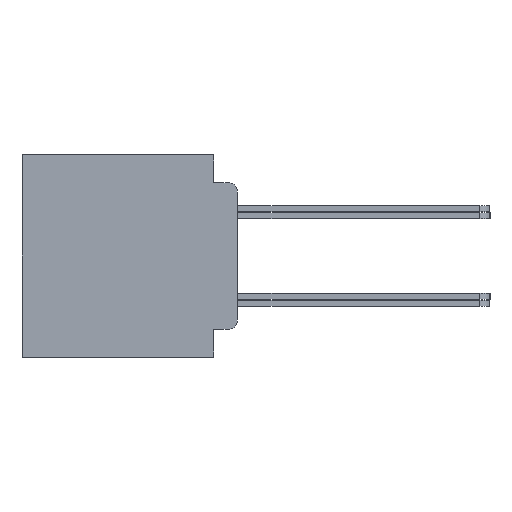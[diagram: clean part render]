
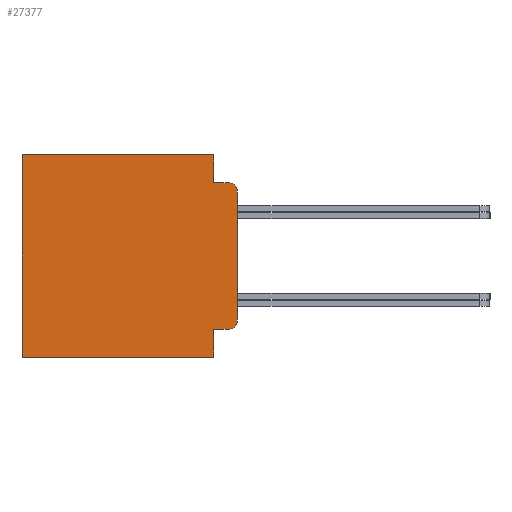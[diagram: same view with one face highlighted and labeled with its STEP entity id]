
A CAD part, left-side view. The second image highlights one B-rep face of the part: STEP entity #27377.
In plain terms, the highlighted planar face has unit normal (-1, 0, 0).
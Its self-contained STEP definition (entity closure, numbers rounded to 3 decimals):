
#7 = VECTOR ( 'NONE', #24448, 1000. ) ;
#81 = CARTESIAN_POINT ( 'NONE',  ( -67.462, 1.295, -3.975 ) ) ;
#483 = VECTOR ( 'NONE', #7830, 1000. ) ;
#488 = ORIENTED_EDGE ( 'NONE', *, *, #22660, .F. ) ;
#946 = CARTESIAN_POINT ( 'NONE',  ( -67.462, 1.295, 3.975 ) ) ;
#1349 = VERTEX_POINT ( 'NONE', #946 ) ;
#1494 = CARTESIAN_POINT ( 'NONE',  ( -67.462, 0., 3.467 ) ) ;
#2006 = EDGE_CURVE ( 'NONE', #25729, #3669, #11912, .T. ) ;
#2063 = LINE ( 'NONE', #21804, #12012 ) ;
#2272 = CARTESIAN_POINT ( 'NONE',  ( -67.462, 11.684, 5.486 ) ) ;
#2387 = AXIS2_PLACEMENT_3D ( 'NONE', #2771, #26645, #26544 ) ;
#2401 = DIRECTION ( 'NONE',  ( 0., 1., 0. ) ) ;
#2612 = VECTOR ( 'NONE', #22150, 1000. ) ;
#2771 = CARTESIAN_POINT ( 'NONE',  ( -67.462, 0., -5.486 ) ) ;
#2920 = ORIENTED_EDGE ( 'NONE', *, *, #2006, .F. ) ;
#3669 = VERTEX_POINT ( 'NONE', #18018 ) ;
#5300 = LINE ( 'NONE', #18003, #5620 ) ;
#5378 = ORIENTED_EDGE ( 'NONE', *, *, #16718, .F. ) ;
#5521 = CARTESIAN_POINT ( 'NONE',  ( -67.462, 0., 5.486 ) ) ;
#5620 = VECTOR ( 'NONE', #15803, 1000. ) ;
#5712 = CARTESIAN_POINT ( 'NONE',  ( -67.462, 1.295, -5.486 ) ) ;
#6053 = VERTEX_POINT ( 'NONE', #17361 ) ;
#6848 = ORIENTED_EDGE ( 'NONE', *, *, #10042, .F. ) ;
#6951 = CARTESIAN_POINT ( 'NONE',  ( -67.462, 1.295, 0. ) ) ;
#7153 = EDGE_CURVE ( 'NONE', #22586, #20848, #27800, .T. ) ;
#7510 = CARTESIAN_POINT ( 'NONE',  ( -67.462, 0., -5.486 ) ) ;
#7711 = LINE ( 'NONE', #9027, #2612 ) ;
#7830 = DIRECTION ( 'NONE',  ( 0., 1., 0. ) ) ;
#8263 = LINE ( 'NONE', #16783, #16468 ) ;
#8578 = DIRECTION ( 'NONE',  ( -1., 0., 0. ) ) ;
#8802 = DIRECTION ( 'NONE',  ( -1., 0., 0. ) ) ;
#9027 = CARTESIAN_POINT ( 'NONE',  ( -67.462, 11.684, -5.486 ) ) ;
#9075 = VERTEX_POINT ( 'NONE', #81 ) ;
#9779 = VERTEX_POINT ( 'NONE', #5712 ) ;
#9884 = EDGE_CURVE ( 'NONE', #19187, #3669, #10281, .T. ) ;
#10042 = EDGE_CURVE ( 'NONE', #9779, #17587, #2063, .T. ) ;
#10281 = CIRCLE ( 'NONE', #15424, 0.508 ) ;
#11272 = ORIENTED_EDGE ( 'NONE', *, *, #13007, .F. ) ;
#11296 = PLANE ( 'NONE',  #2387 ) ;
#11912 = LINE ( 'NONE', #7510, #17011 ) ;
#12012 = VECTOR ( 'NONE', #2401, 1000. ) ;
#12128 = CARTESIAN_POINT ( 'NONE',  ( -67.462, 11.684, -5.486 ) ) ;
#13007 = EDGE_CURVE ( 'NONE', #9075, #9779, #14055, .T. ) ;
#14019 = CARTESIAN_POINT ( 'NONE',  ( -67.462, 0.508, -3.975 ) ) ;
#14055 = LINE ( 'NONE', #6951, #7 ) ;
#15424 = AXIS2_PLACEMENT_3D ( 'NONE', #28138, #8578, #23879 ) ;
#15425 = DIRECTION ( 'NONE',  ( 0., 0., -1. ) ) ;
#15474 = CARTESIAN_POINT ( 'NONE',  ( -67.462, 1.295, 5.486 ) ) ;
#15589 = EDGE_LOOP ( 'NONE', ( #22836, #21873, #2920, #18865, #5378, #488, #21510, #25410, #6848, #11272 ) ) ;
#15727 = FACE_OUTER_BOUND ( 'NONE', #15589, .T. ) ;
#15803 = DIRECTION ( 'NONE',  ( 0., -1., 0. ) ) ;
#16079 = EDGE_CURVE ( 'NONE', #20848, #17587, #7711, .T. ) ;
#16468 = VECTOR ( 'NONE', #19001, 1000. ) ;
#16718 = EDGE_CURVE ( 'NONE', #1349, #6053, #5300, .T. ) ;
#16783 = CARTESIAN_POINT ( 'NONE',  ( -67.462, 1.295, -3.975 ) ) ;
#17011 = VECTOR ( 'NONE', #27172, 1000. ) ;
#17361 = CARTESIAN_POINT ( 'NONE',  ( -67.462, 0.508, 3.975 ) ) ;
#17429 = CARTESIAN_POINT ( 'NONE',  ( -67.462, 0.508, 3.467 ) ) ;
#17587 = VERTEX_POINT ( 'NONE', #12128 ) ;
#18003 = CARTESIAN_POINT ( 'NONE',  ( -67.462, 1.295, 3.975 ) ) ;
#18018 = CARTESIAN_POINT ( 'NONE',  ( -67.462, 0., -3.467 ) ) ;
#18352 = EDGE_CURVE ( 'NONE', #25729, #6053, #19619, .T. ) ;
#18865 = ORIENTED_EDGE ( 'NONE', *, *, #18352, .T. ) ;
#19001 = DIRECTION ( 'NONE',  ( 0., -1., 0. ) ) ;
#19187 = VERTEX_POINT ( 'NONE', #14019 ) ;
#19619 = CIRCLE ( 'NONE', #27380, 0.508 ) ;
#20060 = VECTOR ( 'NONE', #24344, 1000. ) ;
#20848 = VERTEX_POINT ( 'NONE', #2272 ) ;
#21510 = ORIENTED_EDGE ( 'NONE', *, *, #7153, .T. ) ;
#21804 = CARTESIAN_POINT ( 'NONE',  ( -67.462, 0., -5.486 ) ) ;
#21873 = ORIENTED_EDGE ( 'NONE', *, *, #9884, .T. ) ;
#22150 = DIRECTION ( 'NONE',  ( 0., 0., -1. ) ) ;
#22586 = VERTEX_POINT ( 'NONE', #15474 ) ;
#22660 = EDGE_CURVE ( 'NONE', #22586, #1349, #23453, .T. ) ;
#22836 = ORIENTED_EDGE ( 'NONE', *, *, #25766, .T. ) ;
#23453 = LINE ( 'NONE', #26445, #20060 ) ;
#23879 = DIRECTION ( 'NONE',  ( 0., 0., -1. ) ) ;
#24344 = DIRECTION ( 'NONE',  ( 0., 0., -1. ) ) ;
#24448 = DIRECTION ( 'NONE',  ( 0., 0., -1. ) ) ;
#25410 = ORIENTED_EDGE ( 'NONE', *, *, #16079, .T. ) ;
#25729 = VERTEX_POINT ( 'NONE', #1494 ) ;
#25766 = EDGE_CURVE ( 'NONE', #9075, #19187, #8263, .T. ) ;
#26445 = CARTESIAN_POINT ( 'NONE',  ( -67.462, 1.295, 0. ) ) ;
#26544 = DIRECTION ( 'NONE',  ( 0., 0., -1. ) ) ;
#26645 = DIRECTION ( 'NONE',  ( 1., 0., 0. ) ) ;
#27172 = DIRECTION ( 'NONE',  ( 0., 0., -1. ) ) ;
#27377 = ADVANCED_FACE ( 'NONE', ( #15727 ), #11296, .F. ) ;
#27380 = AXIS2_PLACEMENT_3D ( 'NONE', #17429, #8802, #15425 ) ;
#27800 = LINE ( 'NONE', #5521, #483 ) ;
#28138 = CARTESIAN_POINT ( 'NONE',  ( -67.462, 0.508, -3.467 ) ) ;
